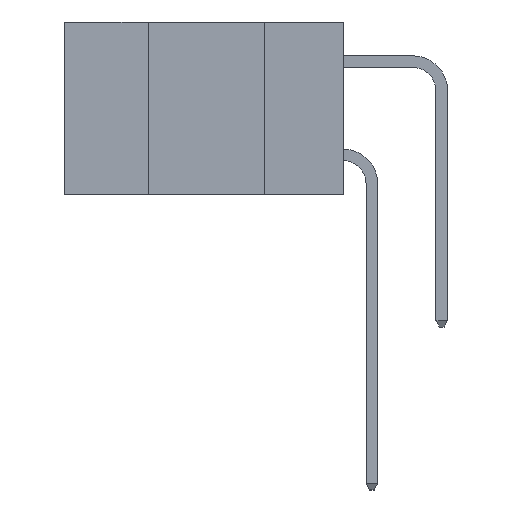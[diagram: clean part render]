
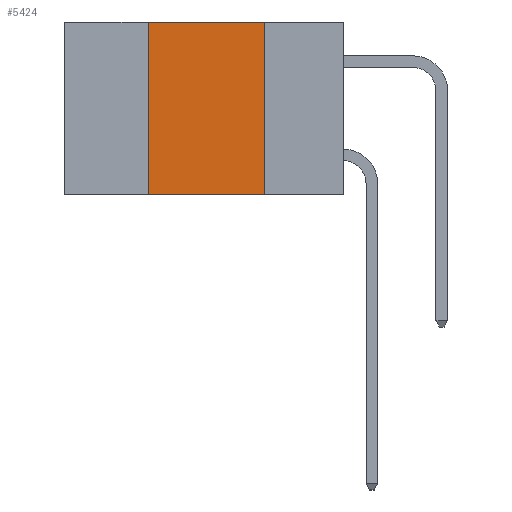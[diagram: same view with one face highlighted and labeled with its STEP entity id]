
A CAD part, left-side view. The second image highlights one B-rep face of the part: STEP entity #5424.
In plain terms, the highlighted planar face has unit normal (-1, 0, 0).
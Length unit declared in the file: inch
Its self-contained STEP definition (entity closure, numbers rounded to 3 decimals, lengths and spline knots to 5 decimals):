
#242 = LINE ( 'NONE', #5755, #6030 ) ;
#463 = CARTESIAN_POINT ( 'NONE',  ( 0., 0.6, -0.37 ) ) ;
#613 = EDGE_LOOP ( 'NONE', ( #10944, #11821, #1559, #1661 ) ) ;
#1355 = EDGE_CURVE ( 'NONE', #2188, #11303, #9878, .T. ) ;
#1559 = ORIENTED_EDGE ( 'NONE', *, *, #1355, .F. ) ;
#1661 = ORIENTED_EDGE ( 'NONE', *, *, #11517, .T. ) ;
#2188 = VERTEX_POINT ( 'NONE', #10853 ) ;
#2451 = VERTEX_POINT ( 'NONE', #6328 ) ;
#2474 = DIRECTION ( 'NONE',  ( 0., -1., 0. ) ) ;
#3649 = EDGE_CURVE ( 'NONE', #10187, #2451, #242, .T. ) ;
#3733 = EDGE_CURVE ( 'NONE', #11303, #10187, #9393, .T. ) ;
#3968 = CARTESIAN_POINT ( 'NONE',  ( 0., 0.6, 0. ) ) ;
#5125 = FACE_OUTER_BOUND ( 'NONE', #613, .T. ) ;
#5424 = ADVANCED_FACE ( 'NONE', ( #5125 ), #10189, .F. ) ;
#5550 = DIRECTION ( 'NONE',  ( 0., 0., -1. ) ) ;
#5744 = CARTESIAN_POINT ( 'NONE',  ( 0., 0.17, 0. ) ) ;
#5755 = CARTESIAN_POINT ( 'NONE',  ( 0., 0.17, -0.37 ) ) ;
#6030 = VECTOR ( 'NONE', #8735, 39.37008 ) ;
#6328 = CARTESIAN_POINT ( 'NONE',  ( 0., 0.17, -0.37 ) ) ;
#7254 = VECTOR ( 'NONE', #9782, 39.37008 ) ;
#7662 = VECTOR ( 'NONE', #2474, 39.37008 ) ;
#8735 = DIRECTION ( 'NONE',  ( 0., 0., -1. ) ) ;
#9046 = DIRECTION ( 'NONE',  ( 1., 0., 0. ) ) ;
#9393 = LINE ( 'NONE', #9449, #11597 ) ;
#9449 = CARTESIAN_POINT ( 'NONE',  ( 0., 0.6, 0. ) ) ;
#9497 = DIRECTION ( 'NONE',  ( 0., -1., 0. ) ) ;
#9782 = DIRECTION ( 'NONE',  ( 0., 0., 1. ) ) ;
#9878 = LINE ( 'NONE', #12491, #7254 ) ;
#10187 = VERTEX_POINT ( 'NONE', #5744 ) ;
#10189 = PLANE ( 'NONE',  #11715 ) ;
#10227 = LINE ( 'NONE', #463, #7662 ) ;
#10755 = CARTESIAN_POINT ( 'NONE',  ( 0., 0.42, 0. ) ) ;
#10853 = CARTESIAN_POINT ( 'NONE',  ( 0., 0.42, -0.37 ) ) ;
#10944 = ORIENTED_EDGE ( 'NONE', *, *, #3649, .F. ) ;
#11303 = VERTEX_POINT ( 'NONE', #10755 ) ;
#11517 = EDGE_CURVE ( 'NONE', #2188, #2451, #10227, .T. ) ;
#11597 = VECTOR ( 'NONE', #9497, 39.37008 ) ;
#11715 = AXIS2_PLACEMENT_3D ( 'NONE', #3968, #9046, #5550 ) ;
#11821 = ORIENTED_EDGE ( 'NONE', *, *, #3733, .F. ) ;
#12491 = CARTESIAN_POINT ( 'NONE',  ( 0., 0.42, -0.37 ) ) ;
